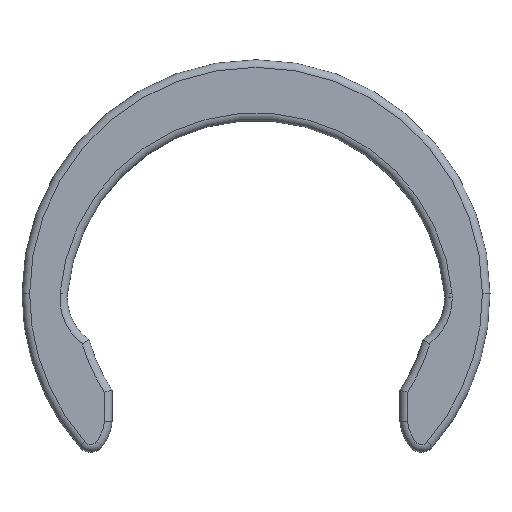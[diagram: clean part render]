
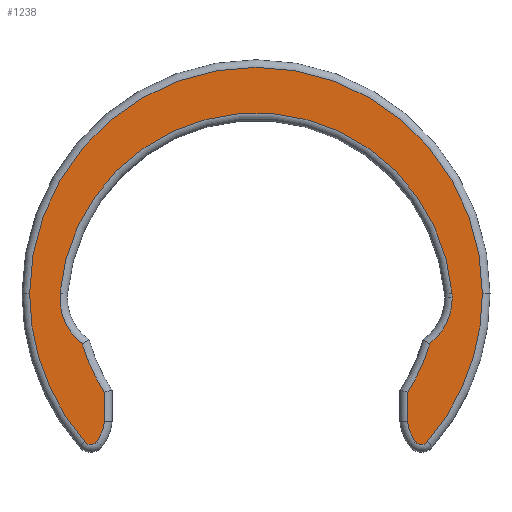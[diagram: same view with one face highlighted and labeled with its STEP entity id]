
A CAD part, top view. The second image highlights one B-rep face of the part: STEP entity #1238.
In plain terms, the highlighted planar face has unit normal (0, 0, 1).
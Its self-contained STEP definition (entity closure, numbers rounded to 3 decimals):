
#2 = DIRECTION ( 'NONE',  ( 0., 0., -1. ) ) ;
#3 = EDGE_CURVE ( 'NONE', #654, #485, #379, .T. ) ;
#19 = CARTESIAN_POINT ( 'NONE',  ( 6.367, -4.051, 0.5 ) ) ;
#24 = EDGE_CURVE ( 'NONE', #1341, #445, #114, .T. ) ;
#27 = AXIS2_PLACEMENT_3D ( 'NONE', #91, #1043, #518 ) ;
#38 = CARTESIAN_POINT ( 'NONE',  ( 0., 0., 0.5 ) ) ;
#50 = DIRECTION ( 'NONE',  ( 1., 0., 0. ) ) ;
#52 = EDGE_CURVE ( 'NONE', #497, #654, #892, .T. ) ;
#57 = CIRCLE ( 'NONE', #149, 7.45 ) ;
#63 = LINE ( 'NONE', #500, #1169 ) ;
#71 = AXIS2_PLACEMENT_3D ( 'NONE', #537, #2, #194 ) ;
#76 = CARTESIAN_POINT ( 'NONE',  ( 0., 0., 0.5 ) ) ;
#91 = CARTESIAN_POINT ( 'NONE',  ( 0., 0., 0.5 ) ) ;
#101 = CARTESIAN_POINT ( 'NONE',  ( 5.717, -1.65, 0.5 ) ) ;
#110 = EDGE_CURVE ( 'NONE', #556, #509, #801, .T. ) ;
#114 = CIRCLE ( 'NONE', #1393, 0.25 ) ;
#125 = VERTEX_POINT ( 'NONE', #442 ) ;
#149 = AXIS2_PLACEMENT_3D ( 'NONE', #76, #504, #407 ) ;
#155 = PLANE ( 'NONE',  #1129 ) ;
#159 = DIRECTION ( 'NONE',  ( 0., 0., 1. ) ) ;
#176 = DIRECTION ( 'NONE',  ( 1., 0., 0. ) ) ;
#178 = VERTEX_POINT ( 'NONE', #503 ) ;
#194 = DIRECTION ( 'NONE',  ( 1., 0., 0. ) ) ;
#202 = EDGE_CURVE ( 'NONE', #559, #497, #644, .T. ) ;
#223 = VERTEX_POINT ( 'NONE', #795 ) ;
#230 = EDGE_CURVE ( 'NONE', #223, #125, #271, .T. ) ;
#235 = EDGE_LOOP ( 'NONE', ( #998, #1000, #332, #281, #553, #725, #651, #1305, #1164, #760, #653, #1093, #868, #677, #880 ) ) ;
#267 = VERTEX_POINT ( 'NONE', #743 ) ;
#271 = CIRCLE ( 'NONE', #1346, 0.25 ) ;
#281 = ORIENTED_EDGE ( 'NONE', *, *, #230, .T. ) ;
#309 = DIRECTION ( 'NONE',  ( 0., 0., 1. ) ) ;
#332 = ORIENTED_EDGE ( 'NONE', *, *, #1100, .T. ) ;
#342 = DIRECTION ( 'NONE',  ( 1., 0., 0. ) ) ;
#349 = DIRECTION ( 'NONE',  ( 0., 0., 1. ) ) ;
#358 = DIRECTION ( 'NONE',  ( 1., 0., 0. ) ) ;
#376 = CIRCLE ( 'NONE', #935, 7.45 ) ;
#379 = CIRCLE ( 'NONE', #446, 1.913 ) ;
#384 = DIRECTION ( 'NONE',  ( 0., -1., 0. ) ) ;
#407 = DIRECTION ( 'NONE',  ( 1., 0., 0. ) ) ;
#442 = CARTESIAN_POINT ( 'NONE',  ( 5.631, -4.878, 0.5 ) ) ;
#445 = VERTEX_POINT ( 'NONE', #1279 ) ;
#446 = AXIS2_PLACEMENT_3D ( 'NONE', #796, #578, #699 ) ;
#450 = DIRECTION ( 'NONE',  ( 0., 0., 1. ) ) ;
#451 = CIRCLE ( 'NONE', #782, 1.387 ) ;
#460 = FACE_OUTER_BOUND ( 'NONE', #235, .T. ) ;
#485 = VERTEX_POINT ( 'NONE', #101 ) ;
#488 = EDGE_CURVE ( 'NONE', #509, #559, #669, .T. ) ;
#497 = VERTEX_POINT ( 'NONE', #521 ) ;
#500 = CARTESIAN_POINT ( 'NONE',  ( 4.988, -4.215, 0.5 ) ) ;
#503 = CARTESIAN_POINT ( 'NONE',  ( 7.45, 0., 0.5 ) ) ;
#504 = DIRECTION ( 'NONE',  ( 0., 0., 1. ) ) ;
#509 = VERTEX_POINT ( 'NONE', #1047 ) ;
#518 = DIRECTION ( 'NONE',  ( 1., 0., 0. ) ) ;
#521 = CARTESIAN_POINT ( 'NONE',  ( 6.449, 0.021, 0.5 ) ) ;
#526 = VERTEX_POINT ( 'NONE', #1304 ) ;
#537 = CARTESIAN_POINT ( 'NONE',  ( -4.543, -0.139, 0.5 ) ) ;
#553 = ORIENTED_EDGE ( 'NONE', *, *, #686, .T. ) ;
#556 = VERTEX_POINT ( 'NONE', #666 ) ;
#559 = VERTEX_POINT ( 'NONE', #768 ) ;
#578 = DIRECTION ( 'NONE',  ( 0., 0., -1. ) ) ;
#584 = AXIS2_PLACEMENT_3D ( 'NONE', #1277, #309, #736 ) ;
#598 = CARTESIAN_POINT ( 'NONE',  ( 6.456, -0.139, 0.5 ) ) ;
#602 = AXIS2_PLACEMENT_3D ( 'NONE', #38, #1215, #342 ) ;
#613 = CARTESIAN_POINT ( 'NONE',  ( -4.988, -3.169, 0.5 ) ) ;
#639 = CARTESIAN_POINT ( 'NONE',  ( -4.988, -4.202, 0.5 ) ) ;
#644 = CIRCLE ( 'NONE', #1080, 6.472 ) ;
#651 = ORIENTED_EDGE ( 'NONE', *, *, #913, .T. ) ;
#653 = ORIENTED_EDGE ( 'NONE', *, *, #110, .T. ) ;
#654 = VERTEX_POINT ( 'NONE', #598 ) ;
#666 = CARTESIAN_POINT ( 'NONE',  ( -4.988, -3.244, 0.5 ) ) ;
#669 = CIRCLE ( 'NONE', #71, 1.913 ) ;
#677 = ORIENTED_EDGE ( 'NONE', *, *, #52, .T. ) ;
#686 = EDGE_CURVE ( 'NONE', #125, #178, #376, .T. ) ;
#691 = CARTESIAN_POINT ( 'NONE',  ( -5.442, -4.714, 0.5 ) ) ;
#699 = DIRECTION ( 'NONE',  ( 1., 0., 0. ) ) ;
#703 = EDGE_CURVE ( 'NONE', #978, #267, #63, .T. ) ;
#725 = ORIENTED_EDGE ( 'NONE', *, *, #1388, .T. ) ;
#736 = DIRECTION ( 'NONE',  ( 1., 0., 0. ) ) ;
#743 = CARTESIAN_POINT ( 'NONE',  ( 4.988, -4.202, 0.5 ) ) ;
#760 = ORIENTED_EDGE ( 'NONE', *, *, #1375, .T. ) ;
#768 = CARTESIAN_POINT ( 'NONE',  ( -6.449, 0.021, 0.5 ) ) ;
#782 = AXIS2_PLACEMENT_3D ( 'NONE', #19, #450, #1078 ) ;
#795 = CARTESIAN_POINT ( 'NONE',  ( 5.239, -4.859, 0.5 ) ) ;
#796 = CARTESIAN_POINT ( 'NONE',  ( 4.543, -0.139, 0.5 ) ) ;
#801 = CIRCLE ( 'NONE', #602, 5.95 ) ;
#807 = AXIS2_PLACEMENT_3D ( 'NONE', #1379, #1158, #1165 ) ;
#811 = EDGE_CURVE ( 'NONE', #485, #978, #1328, .T. ) ;
#824 = LINE ( 'NONE', #613, #950 ) ;
#833 = CARTESIAN_POINT ( 'NONE',  ( 4.988, -3.244, 0.5 ) ) ;
#868 = ORIENTED_EDGE ( 'NONE', *, *, #202, .T. ) ;
#880 = ORIENTED_EDGE ( 'NONE', *, *, #3, .T. ) ;
#881 = CARTESIAN_POINT ( 'NONE',  ( 0., 0., 0.5 ) ) ;
#892 = CIRCLE ( 'NONE', #1175, 1.913 ) ;
#913 = EDGE_CURVE ( 'NONE', #526, #1341, #1111, .T. ) ;
#919 = DIRECTION ( 'NONE',  ( 0., 0., -1. ) ) ;
#927 = DIRECTION ( 'NONE',  ( 1., 0., 0. ) ) ;
#929 = CARTESIAN_POINT ( 'NONE',  ( -5.631, -4.878, 0.5 ) ) ;
#935 = AXIS2_PLACEMENT_3D ( 'NONE', #1021, #159, #50 ) ;
#950 = VECTOR ( 'NONE', #1366, 1000. ) ;
#960 = VERTEX_POINT ( 'NONE', #639 ) ;
#978 = VERTEX_POINT ( 'NONE', #833 ) ;
#998 = ORIENTED_EDGE ( 'NONE', *, *, #811, .T. ) ;
#1000 = ORIENTED_EDGE ( 'NONE', *, *, #703, .T. ) ;
#1019 = DIRECTION ( 'NONE',  ( 0., 0., 1. ) ) ;
#1021 = CARTESIAN_POINT ( 'NONE',  ( 0., 0., 0.5 ) ) ;
#1043 = DIRECTION ( 'NONE',  ( 0., 0., -1. ) ) ;
#1047 = CARTESIAN_POINT ( 'NONE',  ( -5.717, -1.65, 0.5 ) ) ;
#1078 = DIRECTION ( 'NONE',  ( 1., 0., 0. ) ) ;
#1080 = AXIS2_PLACEMENT_3D ( 'NONE', #1130, #919, #358 ) ;
#1093 = ORIENTED_EDGE ( 'NONE', *, *, #488, .T. ) ;
#1100 = EDGE_CURVE ( 'NONE', #267, #223, #451, .T. ) ;
#1111 = CIRCLE ( 'NONE', #807, 7.45 ) ;
#1113 = EDGE_CURVE ( 'NONE', #445, #960, #1266, .T. ) ;
#1123 = CARTESIAN_POINT ( 'NONE',  ( 5.442, -4.714, 0.5 ) ) ;
#1129 = AXIS2_PLACEMENT_3D ( 'NONE', #881, #349, #927 ) ;
#1130 = CARTESIAN_POINT ( 'NONE',  ( 0., -0.522, 0.5 ) ) ;
#1131 = DIRECTION ( 'NONE',  ( 0., 0., 1. ) ) ;
#1145 = DIRECTION ( 'NONE',  ( 0., 0., -1. ) ) ;
#1158 = DIRECTION ( 'NONE',  ( 0., 0., 1. ) ) ;
#1164 = ORIENTED_EDGE ( 'NONE', *, *, #1113, .T. ) ;
#1165 = DIRECTION ( 'NONE',  ( 1., 0., 0. ) ) ;
#1169 = VECTOR ( 'NONE', #384, 1000. ) ;
#1175 = AXIS2_PLACEMENT_3D ( 'NONE', #1344, #1145, #1362 ) ;
#1215 = DIRECTION ( 'NONE',  ( 0., 0., -1. ) ) ;
#1223 = DIRECTION ( 'NONE',  ( 1., 0., 0. ) ) ;
#1238 = ADVANCED_FACE ( 'NONE', ( #460 ), #155, .T. ) ;
#1266 = CIRCLE ( 'NONE', #584, 1.387 ) ;
#1277 = CARTESIAN_POINT ( 'NONE',  ( -6.367, -4.051, 0.5 ) ) ;
#1279 = CARTESIAN_POINT ( 'NONE',  ( -5.239, -4.859, 0.5 ) ) ;
#1304 = CARTESIAN_POINT ( 'NONE',  ( -7.45, 0., 0.5 ) ) ;
#1305 = ORIENTED_EDGE ( 'NONE', *, *, #24, .T. ) ;
#1328 = CIRCLE ( 'NONE', #27, 5.95 ) ;
#1341 = VERTEX_POINT ( 'NONE', #929 ) ;
#1344 = CARTESIAN_POINT ( 'NONE',  ( 4.543, -0.139, 0.5 ) ) ;
#1346 = AXIS2_PLACEMENT_3D ( 'NONE', #1123, #1019, #1223 ) ;
#1362 = DIRECTION ( 'NONE',  ( 1., 0., 0. ) ) ;
#1366 = DIRECTION ( 'NONE',  ( 0., 1., 0. ) ) ;
#1375 = EDGE_CURVE ( 'NONE', #960, #556, #824, .T. ) ;
#1379 = CARTESIAN_POINT ( 'NONE',  ( 0., 0., 0.5 ) ) ;
#1388 = EDGE_CURVE ( 'NONE', #178, #526, #57, .T. ) ;
#1393 = AXIS2_PLACEMENT_3D ( 'NONE', #691, #1131, #176 ) ;
